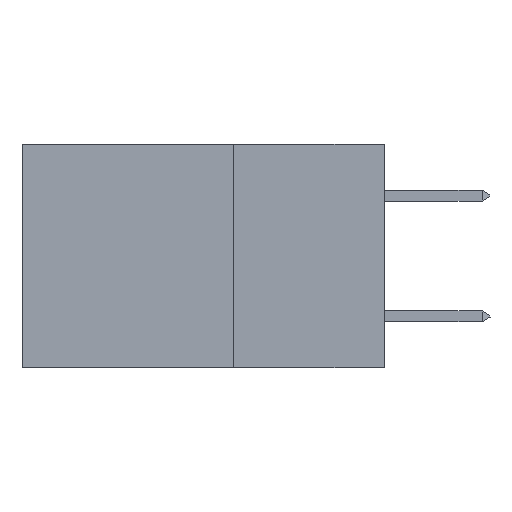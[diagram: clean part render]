
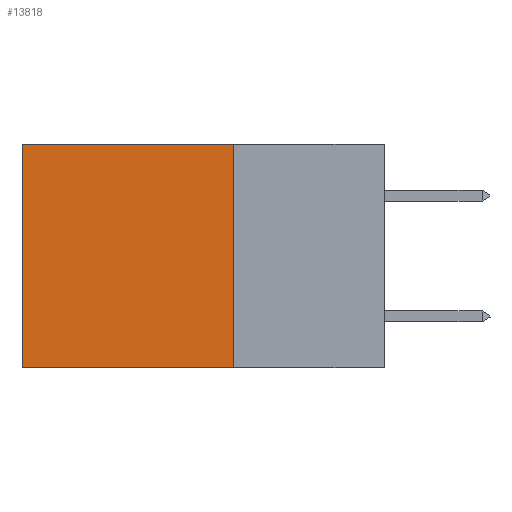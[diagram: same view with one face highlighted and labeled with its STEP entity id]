
A CAD part, left-side view. The second image highlights one B-rep face of the part: STEP entity #13818.
In plain terms, the highlighted planar face has unit normal (-1, 0, 0).
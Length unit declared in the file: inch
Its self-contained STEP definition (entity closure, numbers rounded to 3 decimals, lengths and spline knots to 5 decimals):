
#363 = LINE ( 'NONE', #14718, #7162 ) ;
#876 = VERTEX_POINT ( 'NONE', #15705 ) ;
#1184 = VERTEX_POINT ( 'NONE', #8852 ) ;
#1763 = CARTESIAN_POINT ( 'NONE',  ( 0.2875, 0.25, 0. ) ) ;
#1856 = EDGE_CURVE ( 'NONE', #3547, #876, #14171, .T. ) ;
#3120 = DIRECTION ( 'NONE',  ( 1., 0., 0. ) ) ;
#3155 = LINE ( 'NONE', #13551, #13953 ) ;
#3547 = VERTEX_POINT ( 'NONE', #15038 ) ;
#4284 = EDGE_CURVE ( 'NONE', #1184, #876, #363, .T. ) ;
#4366 = CARTESIAN_POINT ( 'NONE',  ( 0.2875, 0.6, 0. ) ) ;
#4750 = VECTOR ( 'NONE', #11123, 39.37008 ) ;
#5867 = DIRECTION ( 'NONE',  ( 0., 0., -1. ) ) ;
#7162 = VECTOR ( 'NONE', #14738, 39.37008 ) ;
#7762 = FACE_OUTER_BOUND ( 'NONE', #18027, .T. ) ;
#8411 = LINE ( 'NONE', #15424, #4750 ) ;
#8852 = CARTESIAN_POINT ( 'NONE',  ( 0.2875, 0.25, -0.37 ) ) ;
#8933 = VERTEX_POINT ( 'NONE', #17611 ) ;
#10027 = PLANE ( 'NONE',  #11148 ) ;
#11123 = DIRECTION ( 'NONE',  ( 0., 0., -1. ) ) ;
#11148 = AXIS2_PLACEMENT_3D ( 'NONE', #1763, #3120, #12967 ) ;
#11560 = ORIENTED_EDGE ( 'NONE', *, *, #16417, .T. ) ;
#12967 = DIRECTION ( 'NONE',  ( 0., 0., -1. ) ) ;
#13127 = EDGE_CURVE ( 'NONE', #8933, #1184, #8411, .T. ) ;
#13551 = CARTESIAN_POINT ( 'NONE',  ( 0.2875, 0.25, 0. ) ) ;
#13616 = DIRECTION ( 'NONE',  ( 0., 1., 0. ) ) ;
#13818 = ADVANCED_FACE ( 'NONE', ( #7762 ), #10027, .F. ) ;
#13836 = ORIENTED_EDGE ( 'NONE', *, *, #13127, .F. ) ;
#13953 = VECTOR ( 'NONE', #13616, 39.37008 ) ;
#14171 = LINE ( 'NONE', #4366, #17505 ) ;
#14307 = ORIENTED_EDGE ( 'NONE', *, *, #4284, .F. ) ;
#14718 = CARTESIAN_POINT ( 'NONE',  ( 0.2875, 0.25, -0.37 ) ) ;
#14738 = DIRECTION ( 'NONE',  ( 0., 1., 0. ) ) ;
#15038 = CARTESIAN_POINT ( 'NONE',  ( 0.2875, 0.6, 0. ) ) ;
#15424 = CARTESIAN_POINT ( 'NONE',  ( 0.2875, 0.25, 0. ) ) ;
#15705 = CARTESIAN_POINT ( 'NONE',  ( 0.2875, 0.6, -0.37 ) ) ;
#16304 = ORIENTED_EDGE ( 'NONE', *, *, #1856, .T. ) ;
#16417 = EDGE_CURVE ( 'NONE', #8933, #3547, #3155, .T. ) ;
#17505 = VECTOR ( 'NONE', #5867, 39.37008 ) ;
#17611 = CARTESIAN_POINT ( 'NONE',  ( 0.2875, 0.25, 0. ) ) ;
#18027 = EDGE_LOOP ( 'NONE', ( #16304, #14307, #13836, #11560 ) ) ;
